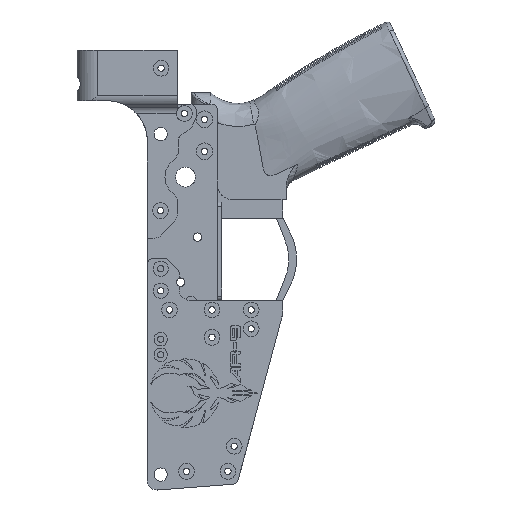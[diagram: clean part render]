
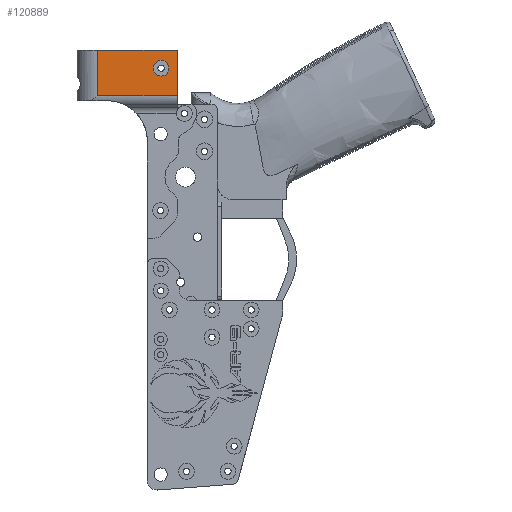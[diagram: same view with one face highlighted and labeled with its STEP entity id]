
A CAD part, left-side view. The second image highlights one B-rep face of the part: STEP entity #120889.
In plain terms, the highlighted planar face has unit normal (-1, 0, 0).
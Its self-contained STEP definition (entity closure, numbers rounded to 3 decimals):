
#4332 = CARTESIAN_POINT ( 'NONE',  ( -25., -22.502, 2.734 ) ) ;
#11318 = AXIS2_PLACEMENT_3D ( 'NONE', #65123, #122020, #19313 ) ;
#11696 = ORIENTED_EDGE ( 'NONE', *, *, #72654, .T. ) ;
#19313 = DIRECTION ( 'NONE',  ( 0., 0., -1. ) ) ;
#20027 = FACE_BOUND ( 'NONE', #76324, .T. ) ;
#24909 = EDGE_CURVE ( 'NONE', #130473, #102278, #126777, .T. ) ;
#36248 = ORIENTED_EDGE ( 'NONE', *, *, #62503, .T. ) ;
#38437 = ORIENTED_EDGE ( 'NONE', *, *, #57407, .T. ) ;
#39622 = CIRCLE ( 'NONE', #141114, 3.75 ) ;
#44227 = CARTESIAN_POINT ( 'NONE',  ( -25., -22.502, 6.484 ) ) ;
#46537 = DIRECTION ( 'NONE',  ( 0., 0., -1. ) ) ;
#48542 = CARTESIAN_POINT ( 'NONE',  ( -25., -22.502, 2.734 ) ) ;
#49098 = CARTESIAN_POINT ( 'NONE',  ( -25., -30.202, -10.291 ) ) ;
#51153 = ORIENTED_EDGE ( 'NONE', *, *, #77502, .T. ) ;
#57127 = LINE ( 'NONE', #67495, #91446 ) ;
#57407 = EDGE_CURVE ( 'NONE', #57505, #64057, #140665, .T. ) ;
#57505 = VERTEX_POINT ( 'NONE', #87404 ) ;
#62503 = EDGE_CURVE ( 'NONE', #119897, #57505, #67234, .T. ) ;
#64057 = VERTEX_POINT ( 'NONE', #49098 ) ;
#65123 = CARTESIAN_POINT ( 'NONE',  ( -25., -36.779, -288600.29 ) ) ;
#67234 = LINE ( 'NONE', #90160, #81310 ) ;
#67495 = CARTESIAN_POINT ( 'NONE',  ( -25., -36.779, 11.224 ) ) ;
#72654 = EDGE_CURVE ( 'NONE', #90229, #119897, #57127, .T. ) ;
#75591 = DIRECTION ( 'NONE',  ( 0., -1., 0. ) ) ;
#76324 = EDGE_LOOP ( 'NONE', ( #120980, #104995 ) ) ;
#77502 = EDGE_CURVE ( 'NONE', #64057, #90229, #119115, .T. ) ;
#81310 = VECTOR ( 'NONE', #46537, 1000. ) ;
#83422 = DIRECTION ( 'NONE',  ( -1., 0., 0. ) ) ;
#84751 = EDGE_LOOP ( 'NONE', ( #36248, #38437, #51153, #11696 ) ) ;
#85856 = CARTESIAN_POINT ( 'NONE',  ( -25., -30.202, -14.306 ) ) ;
#87404 = CARTESIAN_POINT ( 'NONE',  ( -25., 7.678, -10.291 ) ) ;
#90160 = CARTESIAN_POINT ( 'NONE',  ( -25., 7.678, -12.776 ) ) ;
#90229 = VERTEX_POINT ( 'NONE', #122444 ) ;
#91446 = VECTOR ( 'NONE', #145863, 1000. ) ;
#92405 = CARTESIAN_POINT ( 'NONE',  ( -25., 7.678, 11.224 ) ) ;
#95091 = DIRECTION ( 'NONE',  ( -1., 0., 0. ) ) ;
#101741 = EDGE_CURVE ( 'NONE', #102278, #130473, #39622, .T. ) ;
#102278 = VERTEX_POINT ( 'NONE', #136188 ) ;
#103666 = VECTOR ( 'NONE', #141307, 1000. ) ;
#104732 = DIRECTION ( 'NONE',  ( 0., 0., 1. ) ) ;
#104995 = ORIENTED_EDGE ( 'NONE', *, *, #101741, .F. ) ;
#111597 = VECTOR ( 'NONE', #75591, 1000. ) ;
#114515 = DIRECTION ( 'NONE',  ( 0., 0., 1. ) ) ;
#119115 = LINE ( 'NONE', #85856, #103666 ) ;
#119897 = VERTEX_POINT ( 'NONE', #92405 ) ;
#120569 = FACE_OUTER_BOUND ( 'NONE', #84751, .T. ) ;
#120889 = ADVANCED_FACE ( 'NONE', ( #20027, #120569 ), #134571, .F. ) ;
#120980 = ORIENTED_EDGE ( 'NONE', *, *, #24909, .F. ) ;
#122020 = DIRECTION ( 'NONE',  ( 1., 0., 0. ) ) ;
#122444 = CARTESIAN_POINT ( 'NONE',  ( -25., -30.202, 11.224 ) ) ;
#126777 = CIRCLE ( 'NONE', #145635, 3.75 ) ;
#130473 = VERTEX_POINT ( 'NONE', #44227 ) ;
#131771 = CARTESIAN_POINT ( 'NONE',  ( -25., -36.779, -10.291 ) ) ;
#134571 = PLANE ( 'NONE',  #11318 ) ;
#136188 = CARTESIAN_POINT ( 'NONE',  ( -25., -22.502, -1.016 ) ) ;
#140665 = LINE ( 'NONE', #131771, #111597 ) ;
#141114 = AXIS2_PLACEMENT_3D ( 'NONE', #4332, #83422, #114515 ) ;
#141307 = DIRECTION ( 'NONE',  ( 0., 0., 1. ) ) ;
#145635 = AXIS2_PLACEMENT_3D ( 'NONE', #48542, #95091, #104732 ) ;
#145863 = DIRECTION ( 'NONE',  ( 0., 1., 0. ) ) ;
